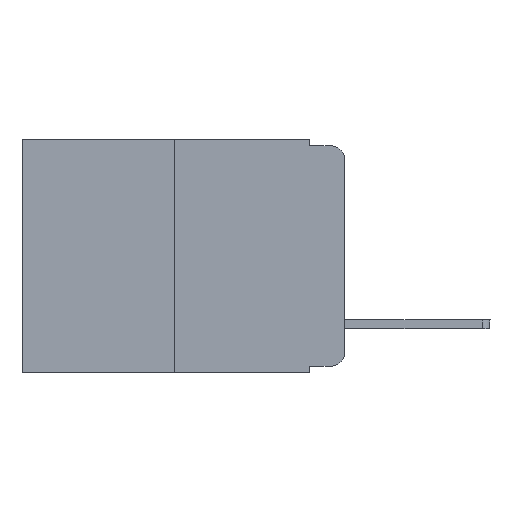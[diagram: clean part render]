
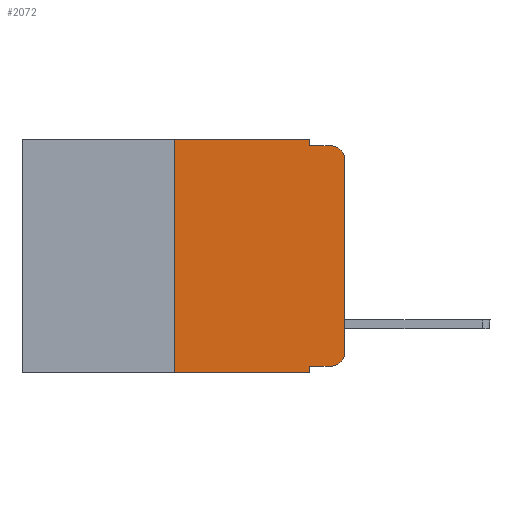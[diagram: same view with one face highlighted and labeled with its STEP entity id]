
A CAD part, left-side view. The second image highlights one B-rep face of the part: STEP entity #2072.
In plain terms, the highlighted planar face has unit normal (-1, 0, 0).
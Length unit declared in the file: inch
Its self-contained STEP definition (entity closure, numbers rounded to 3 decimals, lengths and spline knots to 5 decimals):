
#161 = VERTEX_POINT ( 'NONE', #18716 ) ;
#835 = CARTESIAN_POINT ( 'NONE',  ( 0., 0.051, 0. ) ) ;
#860 = EDGE_CURVE ( 'NONE', #15868, #5554, #5157, .T. ) ;
#898 = CARTESIAN_POINT ( 'NONE',  ( 0., 0.051, 0. ) ) ;
#948 = EDGE_CURVE ( 'NONE', #7613, #5971, #2245, .T. ) ;
#1410 = FACE_OUTER_BOUND ( 'NONE', #14362, .T. ) ;
#1517 = CARTESIAN_POINT ( 'NONE',  ( 0., 0.473, -0.343 ) ) ;
#1867 = ORIENTED_EDGE ( 'NONE', *, *, #2576, .T. ) ;
#2072 = ADVANCED_FACE ( 'NONE', ( #1410 ), #19077, .F. ) ;
#2197 = LINE ( 'NONE', #835, #19013 ) ;
#2209 = LINE ( 'NONE', #9532, #6169 ) ;
#2245 = LINE ( 'NONE', #16731, #16404 ) ;
#2576 = EDGE_CURVE ( 'NONE', #18950, #2760, #6891, .T. ) ;
#2608 = DIRECTION ( 'NONE',  ( 0., -1., 0. ) ) ;
#2760 = VERTEX_POINT ( 'NONE', #17554 ) ;
#2864 = ORIENTED_EDGE ( 'NONE', *, *, #4380, .T. ) ;
#3038 = CARTESIAN_POINT ( 'NONE',  ( 0., 0.473, 0. ) ) ;
#3111 = CARTESIAN_POINT ( 'NONE',  ( 0., 0.02, -0.03 ) ) ;
#3138 = DIRECTION ( 'NONE',  ( 0., -1., 0. ) ) ;
#3219 = EDGE_CURVE ( 'NONE', #4476, #17364, #10364, .T. ) ;
#3256 = ORIENTED_EDGE ( 'NONE', *, *, #13121, .F. ) ;
#4124 = CARTESIAN_POINT ( 'NONE',  ( 0., 0.051, -0.333 ) ) ;
#4280 = ORIENTED_EDGE ( 'NONE', *, *, #17953, .T. ) ;
#4380 = EDGE_CURVE ( 'NONE', #6190, #18950, #2209, .T. ) ;
#4408 = CARTESIAN_POINT ( 'NONE',  ( 0., 0.051, -0.01 ) ) ;
#4476 = VERTEX_POINT ( 'NONE', #4124 ) ;
#4489 = DIRECTION ( 'NONE',  ( 0., 0., -1. ) ) ;
#4861 = DIRECTION ( 'NONE',  ( 0., 0., -1. ) ) ;
#4871 = VECTOR ( 'NONE', #13290, 39.37008 ) ;
#5059 = DIRECTION ( 'NONE',  ( 0., 0., 1. ) ) ;
#5157 = LINE ( 'NONE', #13733, #10194 ) ;
#5344 = EDGE_CURVE ( 'NONE', #17364, #6190, #11129, .T. ) ;
#5468 = CARTESIAN_POINT ( 'NONE',  ( 0., 0., -0.313 ) ) ;
#5554 = VERTEX_POINT ( 'NONE', #8854 ) ;
#5856 = DIRECTION ( 'NONE',  ( 1., 0., 0. ) ) ;
#5971 = VERTEX_POINT ( 'NONE', #4408 ) ;
#6169 = VECTOR ( 'NONE', #16600, 39.37008 ) ;
#6190 = VERTEX_POINT ( 'NONE', #5468 ) ;
#6593 = AXIS2_PLACEMENT_3D ( 'NONE', #3111, #18071, #16449 ) ;
#6891 = CIRCLE ( 'NONE', #6593, 0.02 ) ;
#7575 = VECTOR ( 'NONE', #10234, 39.37008 ) ;
#7613 = VERTEX_POINT ( 'NONE', #898 ) ;
#8071 = DIRECTION ( 'NONE',  ( 0., 0., -1. ) ) ;
#8143 = ORIENTED_EDGE ( 'NONE', *, *, #860, .F. ) ;
#8315 = DIRECTION ( 'NONE',  ( -1., 0., 0. ) ) ;
#8736 = CARTESIAN_POINT ( 'NONE',  ( 0., 0.051, -0.333 ) ) ;
#8836 = LINE ( 'NONE', #1517, #4871 ) ;
#8854 = CARTESIAN_POINT ( 'NONE',  ( 0., 0.25, 0. ) ) ;
#9532 = CARTESIAN_POINT ( 'NONE',  ( 0., 0., 0. ) ) ;
#9765 = CARTESIAN_POINT ( 'NONE',  ( 0., 0.02, -0.313 ) ) ;
#10194 = VECTOR ( 'NONE', #5059, 39.37008 ) ;
#10234 = DIRECTION ( 'NONE',  ( 0., -1., 0. ) ) ;
#10364 = LINE ( 'NONE', #8736, #18912 ) ;
#10447 = ORIENTED_EDGE ( 'NONE', *, *, #3219, .T. ) ;
#10622 = EDGE_CURVE ( 'NONE', #5554, #7613, #14012, .T. ) ;
#11027 = DIRECTION ( 'NONE',  ( 0., 0., -1. ) ) ;
#11129 = CIRCLE ( 'NONE', #15133, 0.02 ) ;
#11517 = VECTOR ( 'NONE', #2608, 39.37008 ) ;
#12648 = CARTESIAN_POINT ( 'NONE',  ( 0., 0.473, 0. ) ) ;
#13121 = EDGE_CURVE ( 'NONE', #4476, #161, #2197, .T. ) ;
#13290 = DIRECTION ( 'NONE',  ( 0., -1., 0. ) ) ;
#13652 = AXIS2_PLACEMENT_3D ( 'NONE', #3038, #5856, #4489 ) ;
#13733 = CARTESIAN_POINT ( 'NONE',  ( 0., 0.25, 0. ) ) ;
#14002 = CARTESIAN_POINT ( 'NONE',  ( 0., 0., -0.03 ) ) ;
#14012 = LINE ( 'NONE', #12648, #11517 ) ;
#14362 = EDGE_LOOP ( 'NONE', ( #2864, #1867, #14799, #14637, #17500, #8143, #4280, #3256, #10447, #18366 ) ) ;
#14637 = ORIENTED_EDGE ( 'NONE', *, *, #948, .F. ) ;
#14799 = ORIENTED_EDGE ( 'NONE', *, *, #15836, .F. ) ;
#15133 = AXIS2_PLACEMENT_3D ( 'NONE', #9765, #8315, #11027 ) ;
#15740 = CARTESIAN_POINT ( 'NONE',  ( 0., 0.02, -0.333 ) ) ;
#15836 = EDGE_CURVE ( 'NONE', #5971, #2760, #16529, .T. ) ;
#15868 = VERTEX_POINT ( 'NONE', #16335 ) ;
#16335 = CARTESIAN_POINT ( 'NONE',  ( 0., 0.25, -0.343 ) ) ;
#16404 = VECTOR ( 'NONE', #4861, 39.37008 ) ;
#16449 = DIRECTION ( 'NONE',  ( 0., 0., -1. ) ) ;
#16529 = LINE ( 'NONE', #19038, #7575 ) ;
#16600 = DIRECTION ( 'NONE',  ( 0., 0., 1. ) ) ;
#16731 = CARTESIAN_POINT ( 'NONE',  ( 0., 0.051, 0. ) ) ;
#17364 = VERTEX_POINT ( 'NONE', #15740 ) ;
#17500 = ORIENTED_EDGE ( 'NONE', *, *, #10622, .F. ) ;
#17554 = CARTESIAN_POINT ( 'NONE',  ( 0., 0.02, -0.01 ) ) ;
#17953 = EDGE_CURVE ( 'NONE', #15868, #161, #8836, .T. ) ;
#18071 = DIRECTION ( 'NONE',  ( -1., 0., 0. ) ) ;
#18366 = ORIENTED_EDGE ( 'NONE', *, *, #5344, .T. ) ;
#18716 = CARTESIAN_POINT ( 'NONE',  ( 0., 0.051, -0.343 ) ) ;
#18912 = VECTOR ( 'NONE', #3138, 39.37008 ) ;
#18950 = VERTEX_POINT ( 'NONE', #14002 ) ;
#19013 = VECTOR ( 'NONE', #8071, 39.37008 ) ;
#19038 = CARTESIAN_POINT ( 'NONE',  ( 0., 0.051, -0.01 ) ) ;
#19077 = PLANE ( 'NONE',  #13652 ) ;
